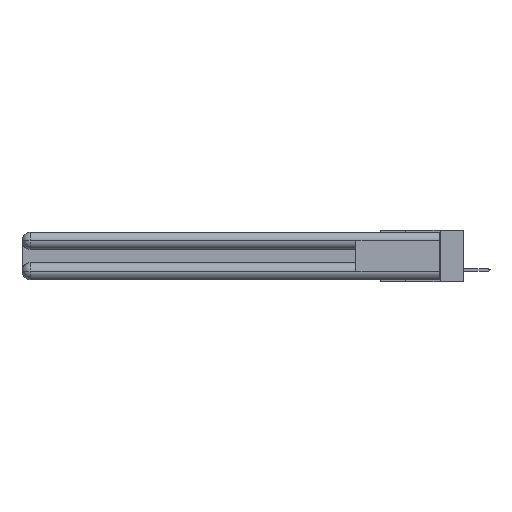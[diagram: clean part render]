
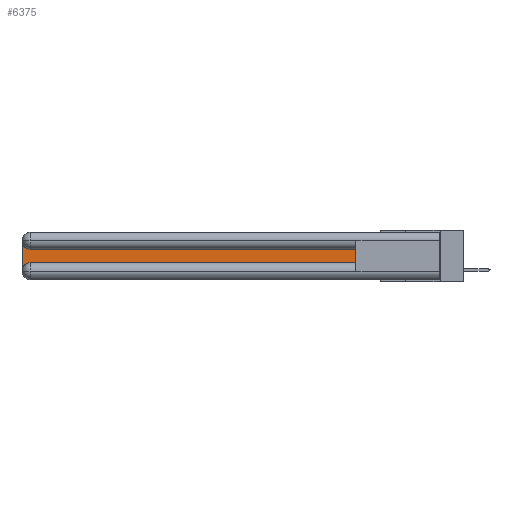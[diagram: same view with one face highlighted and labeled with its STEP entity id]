
A CAD part, left-side view. The second image highlights one B-rep face of the part: STEP entity #6375.
In plain terms, the highlighted planar face has unit normal (-1, 0, 0).
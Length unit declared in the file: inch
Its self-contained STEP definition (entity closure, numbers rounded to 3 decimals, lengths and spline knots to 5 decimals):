
#1545 = ORIENTED_EDGE ( 'NONE', *, *, #5967, .T. ) ;
#2780 = ORIENTED_EDGE ( 'NONE', *, *, #25411, .T. ) ;
#3467 = LINE ( 'NONE', #3469, #32177 ) ;
#3469 = CARTESIAN_POINT ( 'NONE',  ( 0.075, 0.6, -0.2175 ) ) ;
#3862 = CARTESIAN_POINT ( 'NONE',  ( 0.075, 0.6, -0.2175 ) ) ;
#4286 = VECTOR ( 'NONE', #18044, 39.37008 ) ;
#5967 = EDGE_CURVE ( 'NONE', #24759, #33092, #32594, .T. ) ;
#6375 = ADVANCED_FACE ( 'NONE', ( #19195 ), #15518, .F. ) ;
#6870 = DIRECTION ( 'NONE',  ( 1., 0., 0. ) ) ;
#8132 = DIRECTION ( 'NONE',  ( 1., 0., 0. ) ) ;
#8751 = LINE ( 'NONE', #9805, #29849 ) ;
#8936 = VERTEX_POINT ( 'NONE', #31499 ) ;
#9805 = CARTESIAN_POINT ( 'NONE',  ( 0.075, 0.6, -0.1225 ) ) ;
#11111 = AXIS2_PLACEMENT_3D ( 'NONE', #14367, #6870, #24662 ) ;
#11415 = DIRECTION ( 'NONE',  ( 0., 0., -1. ) ) ;
#11762 = CARTESIAN_POINT ( 'NONE',  ( 0.075, 2.94, -0.0625 ) ) ;
#12326 = VERTEX_POINT ( 'NONE', #23392 ) ;
#12404 = DIRECTION ( 'NONE',  ( 0., 1., 0. ) ) ;
#12632 = ORIENTED_EDGE ( 'NONE', *, *, #32455, .T. ) ;
#13041 = CIRCLE ( 'NONE', #30623, 0.06 ) ;
#14367 = CARTESIAN_POINT ( 'NONE',  ( 0.075, 2.94, -0.2775 ) ) ;
#14820 = ORIENTED_EDGE ( 'NONE', *, *, #30111, .T. ) ;
#15518 = PLANE ( 'NONE',  #16451 ) ;
#15691 = ORIENTED_EDGE ( 'NONE', *, *, #18045, .T. ) ;
#16451 = AXIS2_PLACEMENT_3D ( 'NONE', #26366, #8132, #28985 ) ;
#16610 = DIRECTION ( 'NONE',  ( 0., 0., 1. ) ) ;
#17374 = CIRCLE ( 'NONE', #11111, 0.06 ) ;
#18044 = DIRECTION ( 'NONE',  ( 0., 0., -1. ) ) ;
#18045 = EDGE_CURVE ( 'NONE', #29628, #12326, #18828, .T. ) ;
#18811 = ORIENTED_EDGE ( 'NONE', *, *, #24498, .T. ) ;
#18828 = LINE ( 'NONE', #20316, #4286 ) ;
#19195 = FACE_OUTER_BOUND ( 'NONE', #21726, .T. ) ;
#20316 = CARTESIAN_POINT ( 'NONE',  ( 0.075, 3., -0.2175 ) ) ;
#21726 = EDGE_LOOP ( 'NONE', ( #14820, #12632, #15691, #18811, #1545, #2780 ) ) ;
#21764 = CARTESIAN_POINT ( 'NONE',  ( 0.075, 2.94, -0.1225 ) ) ;
#21863 = DIRECTION ( 'NONE',  ( 0., -1., 0. ) ) ;
#21912 = CARTESIAN_POINT ( 'NONE',  ( 0.075, 0.6, -0.2175 ) ) ;
#22503 = CARTESIAN_POINT ( 'NONE',  ( 0.075, 3., -0.0625 ) ) ;
#23392 = CARTESIAN_POINT ( 'NONE',  ( 0.075, 3., -0.2775 ) ) ;
#24498 = EDGE_CURVE ( 'NONE', #12326, #24759, #17374, .T. ) ;
#24662 = DIRECTION ( 'NONE',  ( 0., 0., -1. ) ) ;
#24759 = VERTEX_POINT ( 'NONE', #33227 ) ;
#25251 = VERTEX_POINT ( 'NONE', #21764 ) ;
#25411 = EDGE_CURVE ( 'NONE', #33092, #8936, #3467, .T. ) ;
#26366 = CARTESIAN_POINT ( 'NONE',  ( 0.075, 3., -0.1225 ) ) ;
#28985 = DIRECTION ( 'NONE',  ( 0., 0., -1. ) ) ;
#28996 = VECTOR ( 'NONE', #21863, 39.37008 ) ;
#29628 = VERTEX_POINT ( 'NONE', #22503 ) ;
#29849 = VECTOR ( 'NONE', #12404, 39.37008 ) ;
#30111 = EDGE_CURVE ( 'NONE', #8936, #25251, #8751, .T. ) ;
#30623 = AXIS2_PLACEMENT_3D ( 'NONE', #11762, #32103, #11415 ) ;
#31499 = CARTESIAN_POINT ( 'NONE',  ( 0.075, 0.6, -0.1225 ) ) ;
#32103 = DIRECTION ( 'NONE',  ( 1., 0., 0. ) ) ;
#32177 = VECTOR ( 'NONE', #16610, 39.37008 ) ;
#32455 = EDGE_CURVE ( 'NONE', #25251, #29628, #13041, .T. ) ;
#32594 = LINE ( 'NONE', #3862, #28996 ) ;
#33092 = VERTEX_POINT ( 'NONE', #21912 ) ;
#33227 = CARTESIAN_POINT ( 'NONE',  ( 0.075, 2.94, -0.2175 ) ) ;
